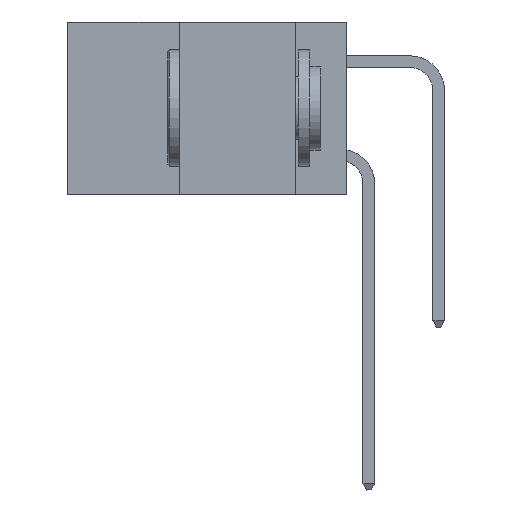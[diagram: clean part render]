
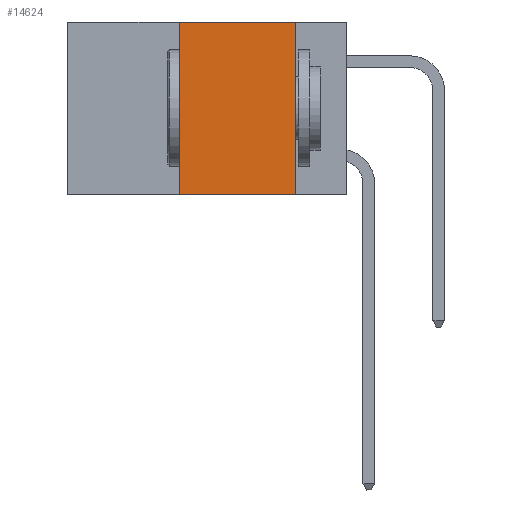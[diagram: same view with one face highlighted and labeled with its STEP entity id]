
A CAD part, left-side view. The second image highlights one B-rep face of the part: STEP entity #14624.
In plain terms, the highlighted planar face has unit normal (-1, 0, 0).
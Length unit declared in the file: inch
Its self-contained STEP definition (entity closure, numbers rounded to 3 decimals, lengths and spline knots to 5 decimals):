
#1201 = CARTESIAN_POINT ( 'NONE',  ( 0., 0.11, 0. ) ) ;
#1844 = AXIS2_PLACEMENT_3D ( 'NONE', #33822, #10984, #16423 ) ;
#2866 = VECTOR ( 'NONE', #11898, 39.37008 ) ;
#5052 = PLANE ( 'NONE',  #1844 ) ;
#6812 = VERTEX_POINT ( 'NONE', #33333 ) ;
#6988 = VERTEX_POINT ( 'NONE', #22854 ) ;
#8640 = VECTOR ( 'NONE', #30969, 39.37008 ) ;
#9000 = ORIENTED_EDGE ( 'NONE', *, *, #33880, .F. ) ;
#9060 = LINE ( 'NONE', #13421, #29905 ) ;
#9078 = LINE ( 'NONE', #18073, #2866 ) ;
#9142 = VECTOR ( 'NONE', #14058, 39.37008 ) ;
#10984 = DIRECTION ( 'NONE',  ( 1., 0., 0. ) ) ;
#11160 = EDGE_CURVE ( 'NONE', #6812, #6988, #11769, .T. ) ;
#11769 = LINE ( 'NONE', #17013, #9142 ) ;
#11898 = DIRECTION ( 'NONE',  ( 0., -1., 0. ) ) ;
#13421 = CARTESIAN_POINT ( 'NONE',  ( 0., 0.11, 0. ) ) ;
#14058 = DIRECTION ( 'NONE',  ( 0., 0., 1. ) ) ;
#14624 = ADVANCED_FACE ( 'NONE', ( #30212 ), #5052, .F. ) ;
#14850 = EDGE_LOOP ( 'NONE', ( #18903, #9000, #25861, #17707 ) ) ;
#16157 = LINE ( 'NONE', #28091, #8640 ) ;
#16423 = DIRECTION ( 'NONE',  ( 0., 0., -1. ) ) ;
#16556 = VERTEX_POINT ( 'NONE', #26660 ) ;
#17013 = CARTESIAN_POINT ( 'NONE',  ( 0., 0.36, 0. ) ) ;
#17379 = EDGE_CURVE ( 'NONE', #6812, #16556, #16157, .T. ) ;
#17707 = ORIENTED_EDGE ( 'NONE', *, *, #17379, .T. ) ;
#18073 = CARTESIAN_POINT ( 'NONE',  ( 0., 0.6, 0. ) ) ;
#18903 = ORIENTED_EDGE ( 'NONE', *, *, #23949, .F. ) ;
#19232 = DIRECTION ( 'NONE',  ( 0., 0., -1. ) ) ;
#22854 = CARTESIAN_POINT ( 'NONE',  ( 0., 0.36, 0. ) ) ;
#23949 = EDGE_CURVE ( 'NONE', #28777, #16556, #9060, .T. ) ;
#25861 = ORIENTED_EDGE ( 'NONE', *, *, #11160, .F. ) ;
#26660 = CARTESIAN_POINT ( 'NONE',  ( 0., 0.11, -0.37 ) ) ;
#28091 = CARTESIAN_POINT ( 'NONE',  ( 0., 0.6, -0.37 ) ) ;
#28777 = VERTEX_POINT ( 'NONE', #1201 ) ;
#29905 = VECTOR ( 'NONE', #19232, 39.37008 ) ;
#30212 = FACE_OUTER_BOUND ( 'NONE', #14850, .T. ) ;
#30969 = DIRECTION ( 'NONE',  ( 0., -1., 0. ) ) ;
#33333 = CARTESIAN_POINT ( 'NONE',  ( 0., 0.36, -0.37 ) ) ;
#33822 = CARTESIAN_POINT ( 'NONE',  ( 0., 0.6, 0. ) ) ;
#33880 = EDGE_CURVE ( 'NONE', #6988, #28777, #9078, .T. ) ;
